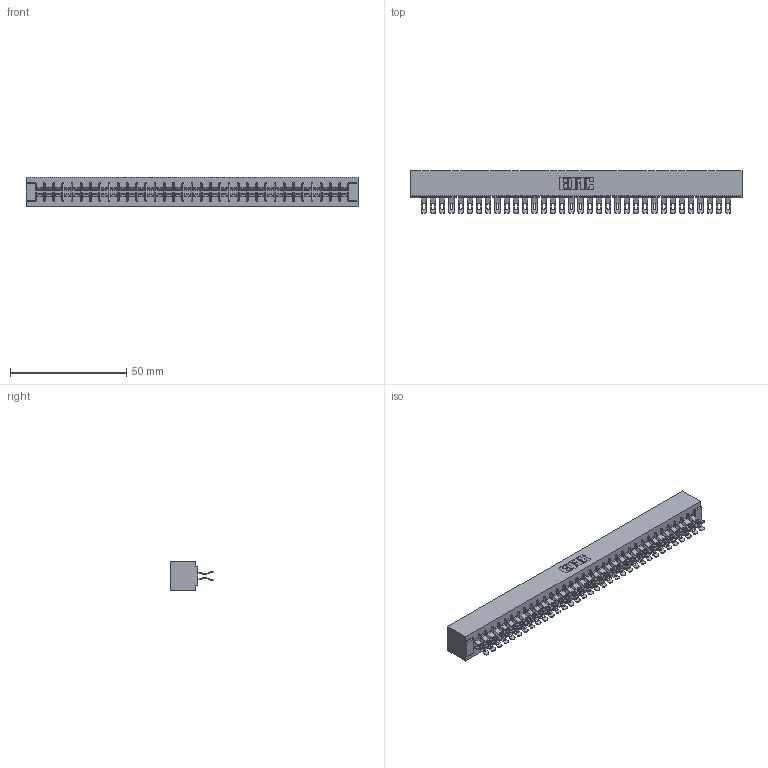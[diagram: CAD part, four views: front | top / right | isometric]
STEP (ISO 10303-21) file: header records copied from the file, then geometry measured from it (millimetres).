
FILE_DESCRIPTION (( 'STEP AP203' ), '1' );
FILE_NAME ('355-068-555-501.STEP', '2019-09-12T17:05:27', ( '' ), ( '' ), 'SwSTEP 2.0', 'SolidWorks 2016', '' );
FILE_SCHEMA (( 'CONFIG_CONTROL_DESIGN' ));
Length unit declared in the file: inch
Products named in the file (3): 305 Part_No Mounting; 355-068-555-501; 305-290-001_555
Assembly tree (69 placements, depth 2):
  355-068-555-501
    305 Part_No Mounting
    305-290-001_555  x68
Bounding box: 142.6 x 18.41 x 12.7 mm (x, y, z)
Volume: 15043.2 mm3; surface area: 21395.6 mm2
Topology: 69 solids, 69 shells, 4596 faces, 13722 edges, 8964 vertices
Faces by surface type: plane 2240, cylinder 2220, sphere 136
Entity records: 38133 total; most frequent: CARTESIAN_POINT 6326, ORIENTED_EDGE 6268, DIRECTION 6118, EDGE_CURVE 3134, LINE 2510, VECTOR 2510, VERTEX_POINT 1996, AXIS2_PLACEMENT_3D 1804
